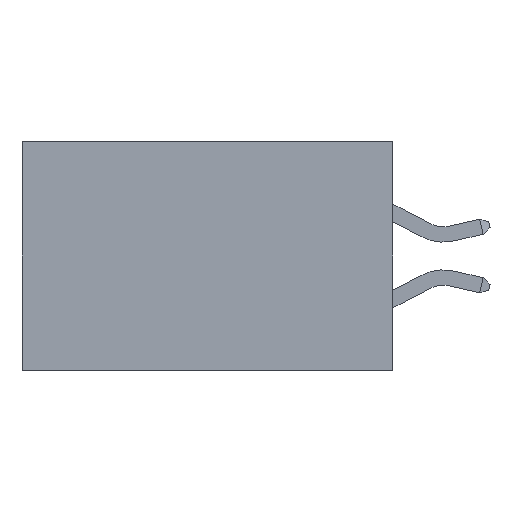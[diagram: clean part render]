
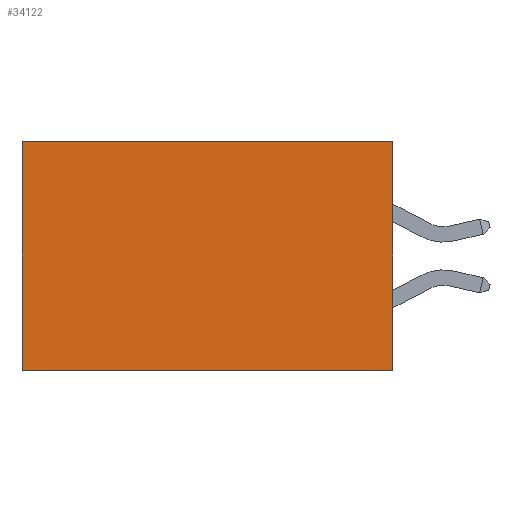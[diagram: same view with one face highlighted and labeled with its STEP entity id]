
A CAD part, left-side view. The second image highlights one B-rep face of the part: STEP entity #34122.
In plain terms, the highlighted planar face has unit normal (-1, 0, 0).
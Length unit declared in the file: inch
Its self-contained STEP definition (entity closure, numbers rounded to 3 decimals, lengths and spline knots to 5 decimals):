
#1174 = DIRECTION ( 'NONE',  ( 0., 0., -1. ) ) ;
#1413 = PLANE ( 'NONE',  #10128 ) ;
#1439 = ORIENTED_EDGE ( 'NONE', *, *, #36518, .F. ) ;
#1947 = CARTESIAN_POINT ( 'NONE',  ( 0.2875, 0., -0.37 ) ) ;
#2217 = CARTESIAN_POINT ( 'NONE',  ( 0.2875, 0.6, 0. ) ) ;
#3077 = VERTEX_POINT ( 'NONE', #7162 ) ;
#4556 = ORIENTED_EDGE ( 'NONE', *, *, #5833, .T. ) ;
#4983 = LINE ( 'NONE', #22069, #18815 ) ;
#5044 = ORIENTED_EDGE ( 'NONE', *, *, #13863, .T. ) ;
#5441 = DIRECTION ( 'NONE',  ( 0., 0., -1. ) ) ;
#5833 = EDGE_CURVE ( 'NONE', #3077, #19174, #9499, .T. ) ;
#7162 = CARTESIAN_POINT ( 'NONE',  ( 0.2875, 0., 0. ) ) ;
#9499 = LINE ( 'NONE', #26216, #10845 ) ;
#10128 = AXIS2_PLACEMENT_3D ( 'NONE', #32524, #15461, #29782 ) ;
#10845 = VECTOR ( 'NONE', #28942, 39.37008 ) ;
#11059 = LINE ( 'NONE', #31484, #16838 ) ;
#11661 = CARTESIAN_POINT ( 'NONE',  ( 0.2875, 0.6, -0.37 ) ) ;
#13212 = EDGE_CURVE ( 'NONE', #3077, #15513, #4983, .T. ) ;
#13863 = EDGE_CURVE ( 'NONE', #19174, #21408, #29459, .T. ) ;
#15461 = DIRECTION ( 'NONE',  ( 1., 0., 0. ) ) ;
#15513 = VERTEX_POINT ( 'NONE', #1947 ) ;
#16838 = VECTOR ( 'NONE', #36665, 39.37008 ) ;
#18815 = VECTOR ( 'NONE', #1174, 39.37008 ) ;
#18954 = CARTESIAN_POINT ( 'NONE',  ( 0.2875, 0.6, 0. ) ) ;
#19174 = VERTEX_POINT ( 'NONE', #18954 ) ;
#21408 = VERTEX_POINT ( 'NONE', #11661 ) ;
#22069 = CARTESIAN_POINT ( 'NONE',  ( 0.2875, 0., 0. ) ) ;
#22528 = FACE_OUTER_BOUND ( 'NONE', #34482, .T. ) ;
#26183 = ORIENTED_EDGE ( 'NONE', *, *, #13212, .F. ) ;
#26216 = CARTESIAN_POINT ( 'NONE',  ( 0.2875, 0., 0. ) ) ;
#28942 = DIRECTION ( 'NONE',  ( 0., 1., 0. ) ) ;
#29459 = LINE ( 'NONE', #2217, #36093 ) ;
#29782 = DIRECTION ( 'NONE',  ( 0., 0., -1. ) ) ;
#31484 = CARTESIAN_POINT ( 'NONE',  ( 0.2875, 0., -0.37 ) ) ;
#32524 = CARTESIAN_POINT ( 'NONE',  ( 0.2875, 0., 0. ) ) ;
#34122 = ADVANCED_FACE ( 'NONE', ( #22528 ), #1413, .F. ) ;
#34482 = EDGE_LOOP ( 'NONE', ( #5044, #1439, #26183, #4556 ) ) ;
#36093 = VECTOR ( 'NONE', #5441, 39.37008 ) ;
#36518 = EDGE_CURVE ( 'NONE', #15513, #21408, #11059, .T. ) ;
#36665 = DIRECTION ( 'NONE',  ( 0., 1., 0. ) ) ;
